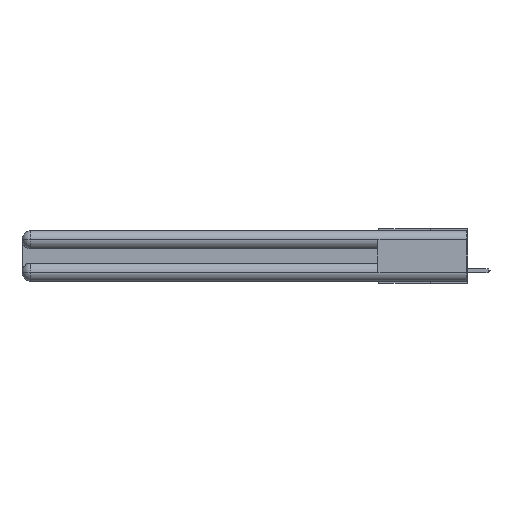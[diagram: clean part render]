
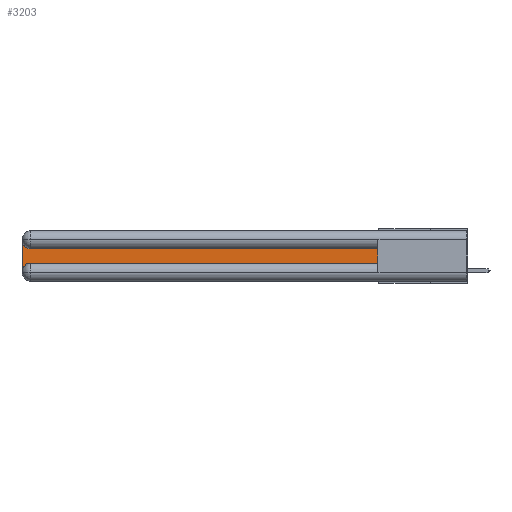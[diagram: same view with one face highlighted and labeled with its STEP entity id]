
A CAD part, left-side view. The second image highlights one B-rep face of the part: STEP entity #3203.
In plain terms, the highlighted planar face has unit normal (-1, 0, 0).
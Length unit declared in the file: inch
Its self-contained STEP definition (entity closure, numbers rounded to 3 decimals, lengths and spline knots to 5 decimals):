
#410 = DIRECTION ( 'NONE',  ( 0., 0., -1. ) ) ;
#748 = CIRCLE ( 'NONE', #27377, 0.06 ) ;
#3203 = ADVANCED_FACE ( 'NONE', ( #19034 ), #10016, .F. ) ;
#3977 = CARTESIAN_POINT ( 'NONE',  ( 0.075, 3., -0.2175 ) ) ;
#4561 = CARTESIAN_POINT ( 'NONE',  ( 0.075, 2.94, -0.2775 ) ) ;
#6090 = ORIENTED_EDGE ( 'NONE', *, *, #14240, .T. ) ;
#6242 = VERTEX_POINT ( 'NONE', #25013 ) ;
#6495 = VERTEX_POINT ( 'NONE', #21132 ) ;
#6641 = EDGE_CURVE ( 'NONE', #6242, #7395, #11883, .T. ) ;
#7352 = VECTOR ( 'NONE', #22216, 39.37008 ) ;
#7395 = VERTEX_POINT ( 'NONE', #9824 ) ;
#7540 = VECTOR ( 'NONE', #10596, 39.37008 ) ;
#8462 = EDGE_CURVE ( 'NONE', #7395, #22765, #748, .T. ) ;
#8796 = VECTOR ( 'NONE', #410, 39.37008 ) ;
#9824 = CARTESIAN_POINT ( 'NONE',  ( 0.075, 2.94, -0.1225 ) ) ;
#9929 = CARTESIAN_POINT ( 'NONE',  ( 0.075, 3., -0.1225 ) ) ;
#10016 = PLANE ( 'NONE',  #19212 ) ;
#10589 = ORIENTED_EDGE ( 'NONE', *, *, #8462, .T. ) ;
#10596 = DIRECTION ( 'NONE',  ( 0., 1., 0. ) ) ;
#11883 = LINE ( 'NONE', #23463, #7540 ) ;
#11896 = ORIENTED_EDGE ( 'NONE', *, *, #16078, .T. ) ;
#12102 = DIRECTION ( 'NONE',  ( 1., 0., 0. ) ) ;
#14240 = EDGE_CURVE ( 'NONE', #22765, #18568, #23530, .T. ) ;
#16078 = EDGE_CURVE ( 'NONE', #6495, #6242, #20993, .T. ) ;
#16192 = CARTESIAN_POINT ( 'NONE',  ( 0.075, 2.94, -0.2175 ) ) ;
#16457 = EDGE_CURVE ( 'NONE', #18568, #17206, #22979, .T. ) ;
#16778 = CARTESIAN_POINT ( 'NONE',  ( 0.075, 3., -0.2775 ) ) ;
#17206 = VERTEX_POINT ( 'NONE', #16192 ) ;
#17321 = AXIS2_PLACEMENT_3D ( 'NONE', #4561, #17480, #19622 ) ;
#17480 = DIRECTION ( 'NONE',  ( 1., 0., 0. ) ) ;
#18322 = ORIENTED_EDGE ( 'NONE', *, *, #16457, .T. ) ;
#18365 = LINE ( 'NONE', #26455, #7352 ) ;
#18568 = VERTEX_POINT ( 'NONE', #16778 ) ;
#19034 = FACE_OUTER_BOUND ( 'NONE', #26769, .T. ) ;
#19212 = AXIS2_PLACEMENT_3D ( 'NONE', #9929, #12102, #27071 ) ;
#19622 = DIRECTION ( 'NONE',  ( 0., 0., -1. ) ) ;
#20989 = DIRECTION ( 'NONE',  ( 0., 0., -1. ) ) ;
#20993 = LINE ( 'NONE', #24442, #23712 ) ;
#21046 = ORIENTED_EDGE ( 'NONE', *, *, #25198, .T. ) ;
#21132 = CARTESIAN_POINT ( 'NONE',  ( 0.075, 0.6, -0.2175 ) ) ;
#22216 = DIRECTION ( 'NONE',  ( 0., -1., 0. ) ) ;
#22765 = VERTEX_POINT ( 'NONE', #27166 ) ;
#22979 = CIRCLE ( 'NONE', #17321, 0.06 ) ;
#23341 = CARTESIAN_POINT ( 'NONE',  ( 0.075, 2.94, -0.0625 ) ) ;
#23463 = CARTESIAN_POINT ( 'NONE',  ( 0.075, 0.6, -0.1225 ) ) ;
#23530 = LINE ( 'NONE', #3977, #8796 ) ;
#23712 = VECTOR ( 'NONE', #24526, 39.37008 ) ;
#23851 = ORIENTED_EDGE ( 'NONE', *, *, #6641, .T. ) ;
#24442 = CARTESIAN_POINT ( 'NONE',  ( 0.075, 0.6, -0.2175 ) ) ;
#24526 = DIRECTION ( 'NONE',  ( 0., 0., 1. ) ) ;
#25013 = CARTESIAN_POINT ( 'NONE',  ( 0.075, 0.6, -0.1225 ) ) ;
#25198 = EDGE_CURVE ( 'NONE', #17206, #6495, #18365, .T. ) ;
#25493 = DIRECTION ( 'NONE',  ( 1., 0., 0. ) ) ;
#26455 = CARTESIAN_POINT ( 'NONE',  ( 0.075, 0.6, -0.2175 ) ) ;
#26769 = EDGE_LOOP ( 'NONE', ( #23851, #10589, #6090, #18322, #21046, #11896 ) ) ;
#27071 = DIRECTION ( 'NONE',  ( 0., 0., -1. ) ) ;
#27166 = CARTESIAN_POINT ( 'NONE',  ( 0.075, 3., -0.0625 ) ) ;
#27377 = AXIS2_PLACEMENT_3D ( 'NONE', #23341, #25493, #20989 ) ;
